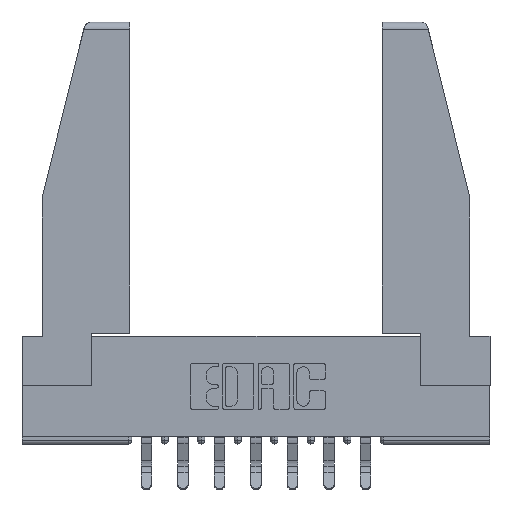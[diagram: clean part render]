
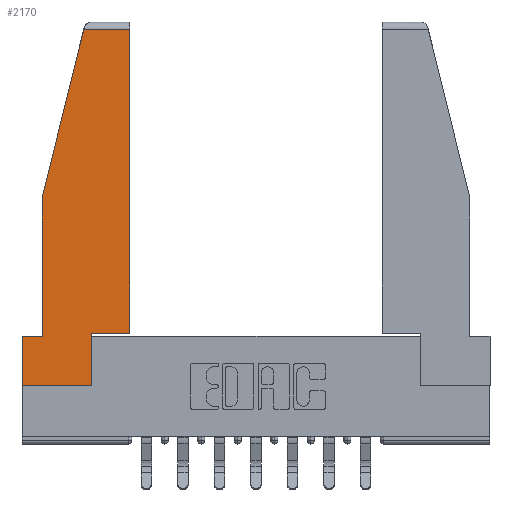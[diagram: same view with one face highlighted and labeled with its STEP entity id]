
A CAD part, top view. The second image highlights one B-rep face of the part: STEP entity #2170.
In plain terms, the highlighted planar face has unit normal (0, 0, 1).
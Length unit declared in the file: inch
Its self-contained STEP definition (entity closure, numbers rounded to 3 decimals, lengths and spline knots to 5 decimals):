
#10 = DIRECTION ( 'NONE',  ( 1., 0., 0. ) ) ;
#124 = LINE ( 'NONE', #3810, #8900 ) ;
#404 = VERTEX_POINT ( 'NONE', #10194 ) ;
#423 = VECTOR ( 'NONE', #6941, 39.37008 ) ;
#595 = VERTEX_POINT ( 'NONE', #6505 ) ;
#626 = VERTEX_POINT ( 'NONE', #766 ) ;
#766 = CARTESIAN_POINT ( 'NONE',  ( 0.2636, 1.52, 0. ) ) ;
#989 = EDGE_CURVE ( 'NONE', #12142, #2660, #124, .T. ) ;
#1407 = DIRECTION ( 'NONE',  ( 1., 0., 0. ) ) ;
#1605 = DIRECTION ( 'NONE',  ( 1., 0., 0. ) ) ;
#2170 = ADVANCED_FACE ( 'NONE', ( #12395 ), #5606, .T. ) ;
#2434 = EDGE_CURVE ( 'NONE', #2957, #4209, #6382, .T. ) ;
#2479 = LINE ( 'NONE', #2795, #5597 ) ;
#2493 = ORIENTED_EDGE ( 'NONE', *, *, #14215, .T. ) ;
#2660 = VERTEX_POINT ( 'NONE', #7145 ) ;
#2795 = CARTESIAN_POINT ( 'NONE',  ( 0., 0.21, 0. ) ) ;
#2957 = VERTEX_POINT ( 'NONE', #9946 ) ;
#3098 = CARTESIAN_POINT ( 'NONE',  ( 0.297, 0., 0. ) ) ;
#3422 = ORIENTED_EDGE ( 'NONE', *, *, #4535, .T. ) ;
#3569 = LINE ( 'NONE', #14496, #12558 ) ;
#3810 = CARTESIAN_POINT ( 'NONE',  ( 0., 0., 0. ) ) ;
#3844 = VECTOR ( 'NONE', #1605, 39.37008 ) ;
#3966 = EDGE_CURVE ( 'NONE', #2660, #6168, #13016, .T. ) ;
#3981 = CARTESIAN_POINT ( 'NONE',  ( 0.271, 1.55, 0. ) ) ;
#4209 = VERTEX_POINT ( 'NONE', #13321 ) ;
#4535 = EDGE_CURVE ( 'NONE', #6168, #595, #6861, .T. ) ;
#5402 = CARTESIAN_POINT ( 'NONE',  ( 0., 0., 0. ) ) ;
#5425 = DIRECTION ( 'NONE',  ( 0., -1., 0. ) ) ;
#5597 = VECTOR ( 'NONE', #7162, 39.37008 ) ;
#5606 = PLANE ( 'NONE',  #7287 ) ;
#5918 = CARTESIAN_POINT ( 'NONE',  ( 0.461, 0.223, 0. ) ) ;
#6168 = VERTEX_POINT ( 'NONE', #8921 ) ;
#6371 = EDGE_LOOP ( 'NONE', ( #8621, #11024, #12105, #10065, #2493, #11690, #10742, #9193, #3422 ) ) ;
#6373 = LINE ( 'NONE', #9141, #13751 ) ;
#6382 = LINE ( 'NONE', #7586, #11486 ) ;
#6495 = DIRECTION ( 'NONE',  ( 0., 1., 0. ) ) ;
#6505 = CARTESIAN_POINT ( 'NONE',  ( 0.461, 0.223, 0. ) ) ;
#6518 = CARTESIAN_POINT ( 'NONE',  ( 0.461, 1.52, 0. ) ) ;
#6570 = DIRECTION ( 'NONE',  ( 0., 0., 1. ) ) ;
#6608 = CARTESIAN_POINT ( 'NONE',  ( 0., 0., 0. ) ) ;
#6767 = EDGE_CURVE ( 'NONE', #9677, #626, #6373, .T. ) ;
#6861 = LINE ( 'NONE', #13821, #3844 ) ;
#6941 = DIRECTION ( 'NONE',  ( 0., 1., 0. ) ) ;
#7145 = CARTESIAN_POINT ( 'NONE',  ( 0.297, 0., 0. ) ) ;
#7162 = DIRECTION ( 'NONE',  ( -1., 0., 0. ) ) ;
#7229 = VECTOR ( 'NONE', #12954, 39.37008 ) ;
#7287 = AXIS2_PLACEMENT_3D ( 'NONE', #5402, #6570, #10 ) ;
#7366 = EDGE_CURVE ( 'NONE', #595, #9677, #9361, .T. ) ;
#7586 = CARTESIAN_POINT ( 'NONE',  ( 0.086, 0.8, 0. ) ) ;
#7768 = VECTOR ( 'NONE', #6495, 39.37008 ) ;
#7786 = DIRECTION ( 'NONE',  ( 0., -1., 0. ) ) ;
#8621 = ORIENTED_EDGE ( 'NONE', *, *, #7366, .T. ) ;
#8900 = VECTOR ( 'NONE', #1407, 39.37008 ) ;
#8921 = CARTESIAN_POINT ( 'NONE',  ( 0.297, 0.223, 0. ) ) ;
#9141 = CARTESIAN_POINT ( 'NONE',  ( 0., 1.52, 0. ) ) ;
#9193 = ORIENTED_EDGE ( 'NONE', *, *, #3966, .T. ) ;
#9361 = LINE ( 'NONE', #5918, #423 ) ;
#9677 = VERTEX_POINT ( 'NONE', #6518 ) ;
#9946 = CARTESIAN_POINT ( 'NONE',  ( 0.086, 0.8, 0. ) ) ;
#10065 = ORIENTED_EDGE ( 'NONE', *, *, #2434, .T. ) ;
#10194 = CARTESIAN_POINT ( 'NONE',  ( 0., 0.21, 0. ) ) ;
#10273 = DIRECTION ( 'NONE',  ( -1., 0., 0. ) ) ;
#10742 = ORIENTED_EDGE ( 'NONE', *, *, #989, .T. ) ;
#11024 = ORIENTED_EDGE ( 'NONE', *, *, #6767, .T. ) ;
#11248 = LINE ( 'NONE', #3981, #7229 ) ;
#11486 = VECTOR ( 'NONE', #5425, 39.37008 ) ;
#11690 = ORIENTED_EDGE ( 'NONE', *, *, #11741, .T. ) ;
#11741 = EDGE_CURVE ( 'NONE', #404, #12142, #3569, .T. ) ;
#12105 = ORIENTED_EDGE ( 'NONE', *, *, #13891, .T. ) ;
#12142 = VERTEX_POINT ( 'NONE', #6608 ) ;
#12395 = FACE_OUTER_BOUND ( 'NONE', #6371, .T. ) ;
#12558 = VECTOR ( 'NONE', #7786, 39.37008 ) ;
#12954 = DIRECTION ( 'NONE',  ( -0.239, -0.971, 0. ) ) ;
#13016 = LINE ( 'NONE', #3098, #7768 ) ;
#13321 = CARTESIAN_POINT ( 'NONE',  ( 0.086, 0.21, 0. ) ) ;
#13751 = VECTOR ( 'NONE', #10273, 39.37008 ) ;
#13821 = CARTESIAN_POINT ( 'NONE',  ( 0.297, 0.223, 0. ) ) ;
#13891 = EDGE_CURVE ( 'NONE', #626, #2957, #11248, .T. ) ;
#14215 = EDGE_CURVE ( 'NONE', #4209, #404, #2479, .T. ) ;
#14496 = CARTESIAN_POINT ( 'NONE',  ( 0., 0.21, 0. ) ) ;
